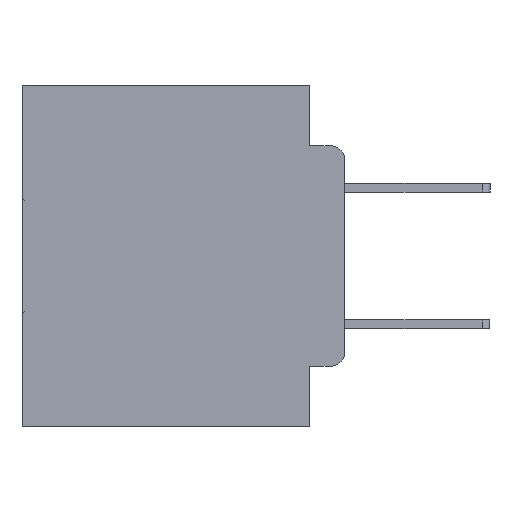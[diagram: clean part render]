
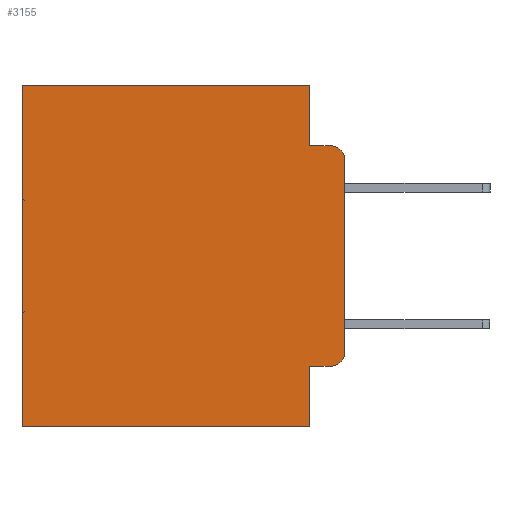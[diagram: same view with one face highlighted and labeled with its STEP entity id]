
A CAD part, left-side view. The second image highlights one B-rep face of the part: STEP entity #3155.
In plain terms, the highlighted planar face has unit normal (-1, 0, 0).
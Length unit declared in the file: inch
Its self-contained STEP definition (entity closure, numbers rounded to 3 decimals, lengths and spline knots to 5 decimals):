
#495 = VECTOR ( 'NONE', #15908, 39.37008 ) ;
#779 = LINE ( 'NONE', #27279, #25727 ) ;
#1290 = CARTESIAN_POINT ( 'NONE',  ( 0.298, 0., 0. ) ) ;
#2463 = VERTEX_POINT ( 'NONE', #12473 ) ;
#2527 = DIRECTION ( 'NONE',  ( 0., 0., -1. ) ) ;
#2630 = PLANE ( 'NONE',  #12686 ) ;
#3058 = CARTESIAN_POINT ( 'NONE',  ( 0.298, 0.02, -0.0885 ) ) ;
#3155 = ADVANCED_FACE ( 'NONE', ( #17281 ), #2630, .F. ) ;
#3866 = DIRECTION ( 'NONE',  ( -1., 0., 0. ) ) ;
#4303 = DIRECTION ( 'NONE',  ( 0., -1., 0. ) ) ;
#4713 = CARTESIAN_POINT ( 'NONE',  ( 0.298, 0.051, 0. ) ) ;
#5829 = CARTESIAN_POINT ( 'NONE',  ( 0.298, 0.473, -0.5 ) ) ;
#5940 = EDGE_CURVE ( 'NONE', #9043, #2463, #28257, .T. ) ;
#6678 = CARTESIAN_POINT ( 'NONE',  ( 0.298, 0.051, -0.5 ) ) ;
#6766 = ORIENTED_EDGE ( 'NONE', *, *, #5940, .T. ) ;
#6799 = LINE ( 'NONE', #9412, #29937 ) ;
#7496 = DIRECTION ( 'NONE',  ( 0., 0., -1. ) ) ;
#8207 = CARTESIAN_POINT ( 'NONE',  ( 0.298, 0.02, -0.3915 ) ) ;
#9043 = VERTEX_POINT ( 'NONE', #21047 ) ;
#9203 = DIRECTION ( 'NONE',  ( 0., 0., -1. ) ) ;
#9412 = CARTESIAN_POINT ( 'NONE',  ( 0.298, 0.051, 0. ) ) ;
#10181 = AXIS2_PLACEMENT_3D ( 'NONE', #18331, #3866, #20698 ) ;
#10250 = ORIENTED_EDGE ( 'NONE', *, *, #19204, .F. ) ;
#10634 = DIRECTION ( 'NONE',  ( 0., 0., -1. ) ) ;
#10741 = CARTESIAN_POINT ( 'NONE',  ( 0.298, 0.051, -0.0885 ) ) ;
#10789 = EDGE_CURVE ( 'NONE', #9043, #24947, #23264, .T. ) ;
#11117 = EDGE_CURVE ( 'NONE', #15115, #26544, #19888, .T. ) ;
#11321 = VECTOR ( 'NONE', #2527, 39.37008 ) ;
#11607 = EDGE_CURVE ( 'NONE', #2463, #22371, #19533, .T. ) ;
#12231 = CARTESIAN_POINT ( 'NONE',  ( 0.298, 0.051, 0. ) ) ;
#12385 = EDGE_CURVE ( 'NONE', #26544, #18931, #22465, .T. ) ;
#12473 = CARTESIAN_POINT ( 'NONE',  ( 0.298, 0.02, -0.4115 ) ) ;
#12685 = AXIS2_PLACEMENT_3D ( 'NONE', #8207, #24922, #10634 ) ;
#12686 = AXIS2_PLACEMENT_3D ( 'NONE', #22695, #23480, #7496 ) ;
#12822 = EDGE_CURVE ( 'NONE', #16216, #19476, #21668, .T. ) ;
#13741 = CARTESIAN_POINT ( 'NONE',  ( 0.298, 0.473, 0. ) ) ;
#14481 = CARTESIAN_POINT ( 'NONE',  ( 0.298, 0., -0.3915 ) ) ;
#14716 = EDGE_CURVE ( 'NONE', #24947, #18931, #779, .T. ) ;
#15115 = VERTEX_POINT ( 'NONE', #4713 ) ;
#15379 = VECTOR ( 'NONE', #20071, 39.37008 ) ;
#15420 = DIRECTION ( 'NONE',  ( 0., 1., 0. ) ) ;
#15442 = EDGE_LOOP ( 'NONE', ( #17347, #19782, #21330, #10250, #24656, #22807, #19194, #24290, #6766, #16119 ) ) ;
#15908 = DIRECTION ( 'NONE',  ( 0., 1., 0. ) ) ;
#16119 = ORIENTED_EDGE ( 'NONE', *, *, #11607, .T. ) ;
#16216 = VERTEX_POINT ( 'NONE', #10741 ) ;
#16542 = DIRECTION ( 'NONE',  ( 0., 0., -1. ) ) ;
#17281 = FACE_OUTER_BOUND ( 'NONE', #15442, .T. ) ;
#17333 = LINE ( 'NONE', #23497, #23635 ) ;
#17347 = ORIENTED_EDGE ( 'NONE', *, *, #30348, .F. ) ;
#17421 = CARTESIAN_POINT ( 'NONE',  ( 0.298, 0.473, 0. ) ) ;
#18142 = VERTEX_POINT ( 'NONE', #20651 ) ;
#18331 = CARTESIAN_POINT ( 'NONE',  ( 0.298, 0.02, -0.1085 ) ) ;
#18732 = CARTESIAN_POINT ( 'NONE',  ( 0.298, 0.051, -0.4115 ) ) ;
#18931 = VERTEX_POINT ( 'NONE', #5829 ) ;
#19194 = ORIENTED_EDGE ( 'NONE', *, *, #14716, .F. ) ;
#19204 = EDGE_CURVE ( 'NONE', #15115, #16216, #6799, .T. ) ;
#19476 = VERTEX_POINT ( 'NONE', #3058 ) ;
#19533 = CIRCLE ( 'NONE', #12685, 0.02 ) ;
#19782 = ORIENTED_EDGE ( 'NONE', *, *, #20799, .T. ) ;
#19888 = LINE ( 'NONE', #1290, #495 ) ;
#20071 = DIRECTION ( 'NONE',  ( 0., -1., 0. ) ) ;
#20651 = CARTESIAN_POINT ( 'NONE',  ( 0.298, 0., -0.1085 ) ) ;
#20698 = DIRECTION ( 'NONE',  ( 0., 0., -1. ) ) ;
#20799 = EDGE_CURVE ( 'NONE', #18142, #19476, #23159, .T. ) ;
#21047 = CARTESIAN_POINT ( 'NONE',  ( 0.298, 0.051, -0.4115 ) ) ;
#21330 = ORIENTED_EDGE ( 'NONE', *, *, #12822, .F. ) ;
#21668 = LINE ( 'NONE', #27155, #15379 ) ;
#22371 = VERTEX_POINT ( 'NONE', #14481 ) ;
#22465 = LINE ( 'NONE', #13741, #23217 ) ;
#22695 = CARTESIAN_POINT ( 'NONE',  ( 0.298, 0., 0. ) ) ;
#22807 = ORIENTED_EDGE ( 'NONE', *, *, #12385, .T. ) ;
#23159 = CIRCLE ( 'NONE', #10181, 0.02 ) ;
#23217 = VECTOR ( 'NONE', #28015, 39.37008 ) ;
#23264 = LINE ( 'NONE', #12231, #11321 ) ;
#23480 = DIRECTION ( 'NONE',  ( 1., 0., 0. ) ) ;
#23497 = CARTESIAN_POINT ( 'NONE',  ( 0.298, 0., 0. ) ) ;
#23635 = VECTOR ( 'NONE', #9203, 39.37008 ) ;
#24290 = ORIENTED_EDGE ( 'NONE', *, *, #10789, .F. ) ;
#24656 = ORIENTED_EDGE ( 'NONE', *, *, #11117, .T. ) ;
#24922 = DIRECTION ( 'NONE',  ( -1., 0., 0. ) ) ;
#24947 = VERTEX_POINT ( 'NONE', #6678 ) ;
#25727 = VECTOR ( 'NONE', #15420, 39.37008 ) ;
#26544 = VERTEX_POINT ( 'NONE', #17421 ) ;
#27155 = CARTESIAN_POINT ( 'NONE',  ( 0.298, 0.051, -0.0885 ) ) ;
#27279 = CARTESIAN_POINT ( 'NONE',  ( 0.298, 0., -0.5 ) ) ;
#28015 = DIRECTION ( 'NONE',  ( 0., 0., -1. ) ) ;
#28257 = LINE ( 'NONE', #18732, #28982 ) ;
#28982 = VECTOR ( 'NONE', #4303, 39.37008 ) ;
#29937 = VECTOR ( 'NONE', #16542, 39.37008 ) ;
#30348 = EDGE_CURVE ( 'NONE', #18142, #22371, #17333, .T. ) ;
